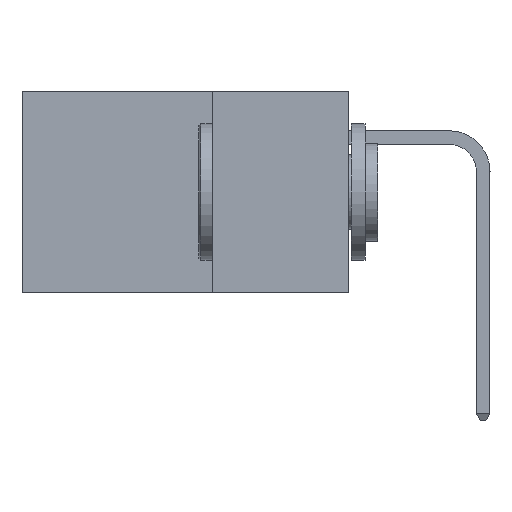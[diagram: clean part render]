
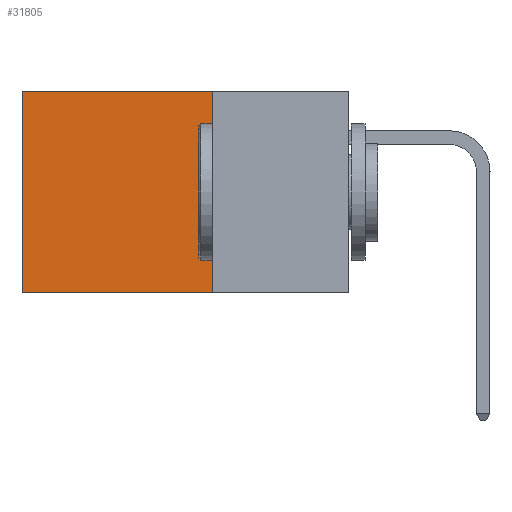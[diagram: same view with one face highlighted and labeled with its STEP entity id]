
A CAD part, left-side view. The second image highlights one B-rep face of the part: STEP entity #31805.
In plain terms, the highlighted planar face has unit normal (-1, 0, 0).
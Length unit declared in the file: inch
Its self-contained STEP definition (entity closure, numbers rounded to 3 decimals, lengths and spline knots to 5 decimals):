
#2272 = CARTESIAN_POINT ( 'NONE',  ( 0.2875, 0.25, 0. ) ) ;
#5149 = EDGE_CURVE ( 'NONE', #11316, #20939, #45240, .T. ) ;
#6445 = ORIENTED_EDGE ( 'NONE', *, *, #15628, .F. ) ;
#8071 = CARTESIAN_POINT ( 'NONE',  ( 0.2875, 0.6, 0. ) ) ;
#8528 = DIRECTION ( 'NONE',  ( 0., 0., -1. ) ) ;
#9254 = EDGE_CURVE ( 'NONE', #31928, #20939, #41166, .T. ) ;
#9902 = VECTOR ( 'NONE', #19908, 39.37008 ) ;
#11316 = VERTEX_POINT ( 'NONE', #21939 ) ;
#11465 = CARTESIAN_POINT ( 'NONE',  ( 0.2875, 0.6, 0. ) ) ;
#11977 = EDGE_LOOP ( 'NONE', ( #13739, #17216, #6445, #30373 ) ) ;
#12443 = DIRECTION ( 'NONE',  ( 0., 1., 0. ) ) ;
#13354 = DIRECTION ( 'NONE',  ( 0., 0., -1. ) ) ;
#13739 = ORIENTED_EDGE ( 'NONE', *, *, #9254, .T. ) ;
#15628 = EDGE_CURVE ( 'NONE', #19099, #11316, #23338, .T. ) ;
#16547 = PLANE ( 'NONE',  #39180 ) ;
#17216 = ORIENTED_EDGE ( 'NONE', *, *, #5149, .F. ) ;
#19099 = VERTEX_POINT ( 'NONE', #48163 ) ;
#19146 = CARTESIAN_POINT ( 'NONE',  ( 0.2875, 0.6, -0.37 ) ) ;
#19908 = DIRECTION ( 'NONE',  ( 0., 0., -1. ) ) ;
#20939 = VERTEX_POINT ( 'NONE', #19146 ) ;
#21939 = CARTESIAN_POINT ( 'NONE',  ( 0.2875, 0.25, -0.37 ) ) ;
#23338 = LINE ( 'NONE', #2272, #23969 ) ;
#23969 = VECTOR ( 'NONE', #13354, 39.37008 ) ;
#24656 = VECTOR ( 'NONE', #12443, 39.37008 ) ;
#29216 = CARTESIAN_POINT ( 'NONE',  ( 0.2875, 0.25, -0.37 ) ) ;
#30373 = ORIENTED_EDGE ( 'NONE', *, *, #41203, .T. ) ;
#31805 = ADVANCED_FACE ( 'NONE', ( #48474 ), #16547, .F. ) ;
#31928 = VERTEX_POINT ( 'NONE', #11465 ) ;
#32301 = CARTESIAN_POINT ( 'NONE',  ( 0.2875, 0.25, 0. ) ) ;
#35562 = CARTESIAN_POINT ( 'NONE',  ( 0.2875, 0.25, 0. ) ) ;
#37539 = LINE ( 'NONE', #32301, #24656 ) ;
#38874 = DIRECTION ( 'NONE',  ( 1., 0., 0. ) ) ;
#39180 = AXIS2_PLACEMENT_3D ( 'NONE', #35562, #38874, #8528 ) ;
#41166 = LINE ( 'NONE', #8071, #9902 ) ;
#41203 = EDGE_CURVE ( 'NONE', #19099, #31928, #37539, .T. ) ;
#41226 = DIRECTION ( 'NONE',  ( 0., 1., 0. ) ) ;
#45240 = LINE ( 'NONE', #29216, #47707 ) ;
#47707 = VECTOR ( 'NONE', #41226, 39.37008 ) ;
#48163 = CARTESIAN_POINT ( 'NONE',  ( 0.2875, 0.25, 0. ) ) ;
#48474 = FACE_OUTER_BOUND ( 'NONE', #11977, .T. ) ;
